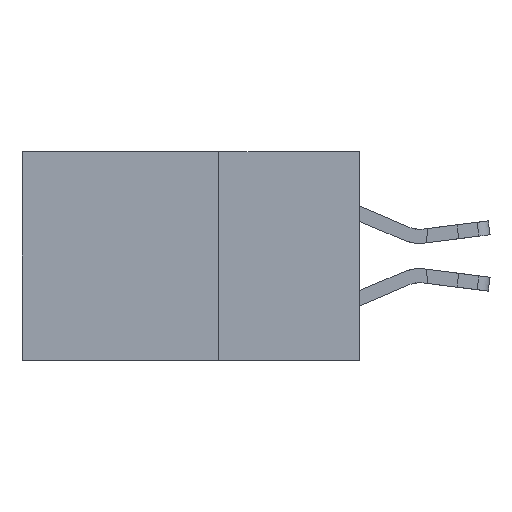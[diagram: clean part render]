
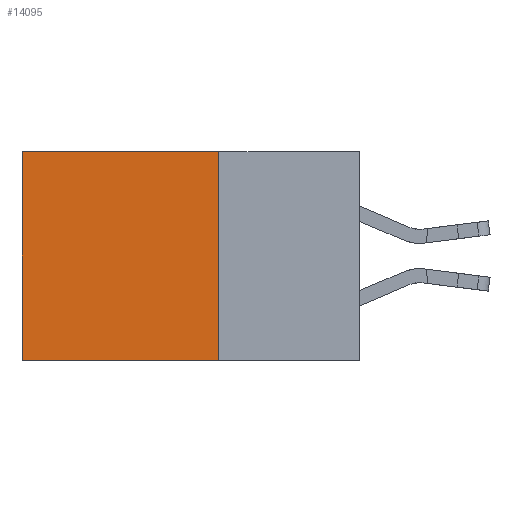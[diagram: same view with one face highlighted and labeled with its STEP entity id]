
A CAD part, left-side view. The second image highlights one B-rep face of the part: STEP entity #14095.
In plain terms, the highlighted planar face has unit normal (-1, 0, 0).
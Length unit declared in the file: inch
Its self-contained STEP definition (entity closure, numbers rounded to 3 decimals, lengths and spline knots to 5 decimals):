
#202 = EDGE_CURVE ( 'NONE', #7735, #2280, #8266, .T. ) ;
#207 = EDGE_CURVE ( 'NONE', #14574, #2280, #15913, .T. ) ;
#920 = FACE_OUTER_BOUND ( 'NONE', #6813, .T. ) ;
#2280 = VERTEX_POINT ( 'NONE', #13911 ) ;
#2577 = ORIENTED_EDGE ( 'NONE', *, *, #3509, .T. ) ;
#3033 = ORIENTED_EDGE ( 'NONE', *, *, #207, .F. ) ;
#3218 = VECTOR ( 'NONE', #16060, 39.37008 ) ;
#3433 = LINE ( 'NONE', #6438, #3218 ) ;
#3463 = CARTESIAN_POINT ( 'NONE',  ( 0.2875, 0.6, 0. ) ) ;
#3509 = EDGE_CURVE ( 'NONE', #6164, #7735, #10666, .T. ) ;
#3948 = CARTESIAN_POINT ( 'NONE',  ( 0.2875, 0.6, 0. ) ) ;
#4162 = ORIENTED_EDGE ( 'NONE', *, *, #202, .T. ) ;
#4831 = CARTESIAN_POINT ( 'NONE',  ( 0.2875, 0.25, 0. ) ) ;
#6164 = VERTEX_POINT ( 'NONE', #6699 ) ;
#6438 = CARTESIAN_POINT ( 'NONE',  ( 0.2875, 0.25, 0. ) ) ;
#6699 = CARTESIAN_POINT ( 'NONE',  ( 0.2875, 0.25, 0. ) ) ;
#6813 = EDGE_LOOP ( 'NONE', ( #4162, #3033, #14001, #2577 ) ) ;
#7506 = CARTESIAN_POINT ( 'NONE',  ( 0.2875, 0.25, -0.37 ) ) ;
#7735 = VERTEX_POINT ( 'NONE', #3948 ) ;
#7981 = CARTESIAN_POINT ( 'NONE',  ( 0.2875, 0.25, 0. ) ) ;
#8266 = LINE ( 'NONE', #3463, #11454 ) ;
#8985 = CARTESIAN_POINT ( 'NONE',  ( 0.2875, 0.25, -0.37 ) ) ;
#10666 = LINE ( 'NONE', #4831, #13655 ) ;
#11454 = VECTOR ( 'NONE', #13019, 39.37008 ) ;
#11738 = DIRECTION ( 'NONE',  ( 0., 1., 0. ) ) ;
#11804 = AXIS2_PLACEMENT_3D ( 'NONE', #7981, #15990, #12129 ) ;
#12129 = DIRECTION ( 'NONE',  ( 0., 0., -1. ) ) ;
#13019 = DIRECTION ( 'NONE',  ( 0., 0., -1. ) ) ;
#13655 = VECTOR ( 'NONE', #14790, 39.37008 ) ;
#13911 = CARTESIAN_POINT ( 'NONE',  ( 0.2875, 0.6, -0.37 ) ) ;
#14001 = ORIENTED_EDGE ( 'NONE', *, *, #15607, .F. ) ;
#14095 = ADVANCED_FACE ( 'NONE', ( #920 ), #17535, .F. ) ;
#14574 = VERTEX_POINT ( 'NONE', #7506 ) ;
#14790 = DIRECTION ( 'NONE',  ( 0., 1., 0. ) ) ;
#15607 = EDGE_CURVE ( 'NONE', #6164, #14574, #3433, .T. ) ;
#15713 = VECTOR ( 'NONE', #11738, 39.37008 ) ;
#15913 = LINE ( 'NONE', #8985, #15713 ) ;
#15990 = DIRECTION ( 'NONE',  ( 1., 0., 0. ) ) ;
#16060 = DIRECTION ( 'NONE',  ( 0., 0., -1. ) ) ;
#17535 = PLANE ( 'NONE',  #11804 ) ;
